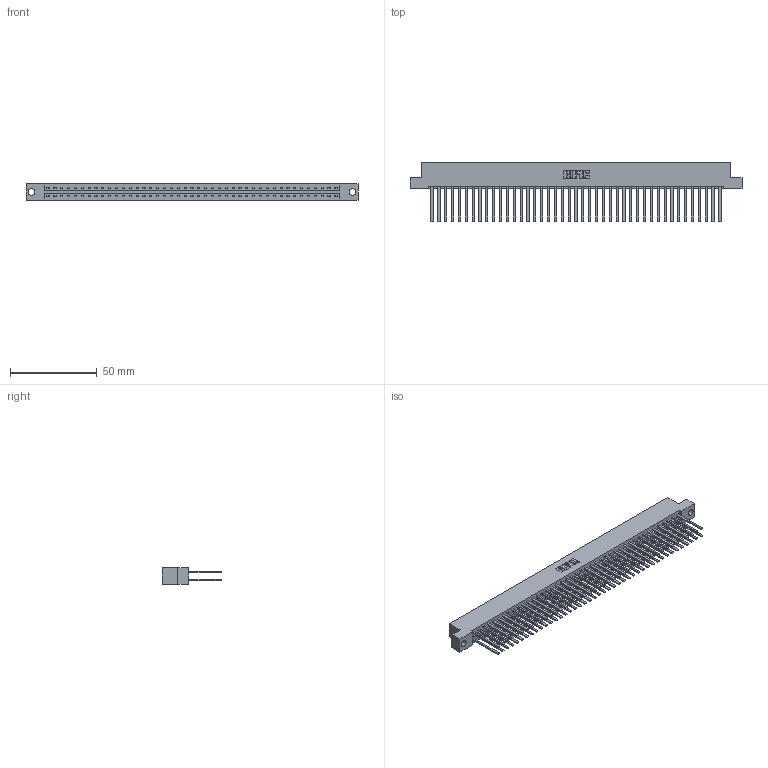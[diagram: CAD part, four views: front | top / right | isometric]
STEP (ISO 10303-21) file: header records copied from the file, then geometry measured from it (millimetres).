
FILE_DESCRIPTION (( 'STEP AP203' ), '1' );
FILE_NAME ('833-086-544-204.STEP', '2020-06-06T03:43:17', ( '' ), ( '' ), 'SwSTEP 2.0', 'SolidWorks 2020', '' );
FILE_SCHEMA (( 'CONFIG_CONTROL_DESIGN' ));
Length unit declared in the file: inch
Products named in the file (3): 833-086-544-204; 345-292-001_345-293-144; 833 Part_Flush - .156 Dia - TH
Assembly tree (87 placements, depth 2):
  833-086-544-204
    833 Part_Flush - .156 Dia - TH
    345-292-001_345-293-144  x86
Bounding box: 191.92 x 34.3 x 9.4 mm (x, y, z)
Volume: 20721.2 mm3; surface area: 28189.4 mm2
Topology: 87 solids, 87 shells, 4070 faces, 12093 edges, 7946 vertices
Faces by surface type: plane 2822, cylinder 1248
Entity records: 27353 total; most frequent: CARTESIAN_POINT 4530, ORIENTED_EDGE 4466, DIRECTION 3865, EDGE_CURVE 2233, LINE 2109, VECTOR 2109, VERTEX_POINT 1486, AXIS2_PLACEMENT_3D 878
